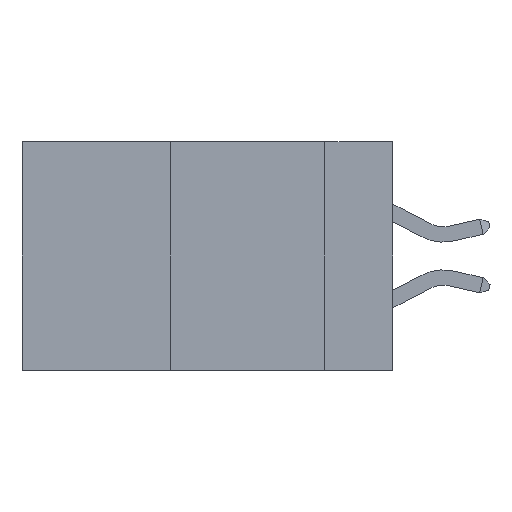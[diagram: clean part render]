
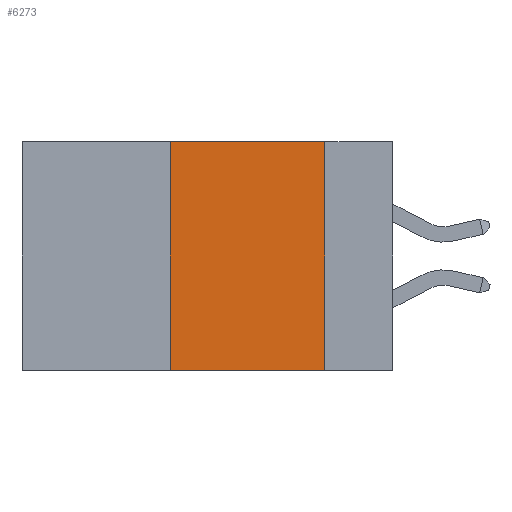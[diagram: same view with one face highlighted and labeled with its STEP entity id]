
A CAD part, left-side view. The second image highlights one B-rep face of the part: STEP entity #6273.
In plain terms, the highlighted planar face has unit normal (-1, 0, 0).
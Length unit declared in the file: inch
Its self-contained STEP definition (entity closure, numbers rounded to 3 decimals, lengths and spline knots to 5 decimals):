
#93 = EDGE_CURVE ( 'NONE', #15959, #1141, #6287, .T. ) ;
#299 = VERTEX_POINT ( 'NONE', #10447 ) ;
#703 = ORIENTED_EDGE ( 'NONE', *, *, #93, .F. ) ;
#957 = EDGE_CURVE ( 'NONE', #299, #5131, #10034, .T. ) ;
#1141 = VERTEX_POINT ( 'NONE', #5222 ) ;
#1357 = DIRECTION ( 'NONE',  ( 0., 0., 1. ) ) ;
#2706 = CARTESIAN_POINT ( 'NONE',  ( 0., 0.11, 0. ) ) ;
#3275 = DIRECTION ( 'NONE',  ( 0., -1., 0. ) ) ;
#3930 = DIRECTION ( 'NONE',  ( 0., 0., -1. ) ) ;
#3969 = CARTESIAN_POINT ( 'NONE',  ( 0., 0.6, 0. ) ) ;
#5131 = VERTEX_POINT ( 'NONE', #12251 ) ;
#5210 = VECTOR ( 'NONE', #16114, 39.37008 ) ;
#5222 = CARTESIAN_POINT ( 'NONE',  ( 0., 0.11, -0.37 ) ) ;
#5848 = VECTOR ( 'NONE', #13717, 39.37008 ) ;
#6216 = CARTESIAN_POINT ( 'NONE',  ( 0., 0.6, 0. ) ) ;
#6273 = ADVANCED_FACE ( 'NONE', ( #15174 ), #6758, .F. ) ;
#6287 = LINE ( 'NONE', #2706, #5848 ) ;
#6758 = PLANE ( 'NONE',  #11987 ) ;
#6806 = DIRECTION ( 'NONE',  ( 1., 0., 0. ) ) ;
#6867 = CARTESIAN_POINT ( 'NONE',  ( 0., 0.36, 0. ) ) ;
#7889 = EDGE_CURVE ( 'NONE', #5131, #15959, #8968, .T. ) ;
#8968 = LINE ( 'NONE', #3969, #5210 ) ;
#9175 = VECTOR ( 'NONE', #3275, 39.37008 ) ;
#10034 = LINE ( 'NONE', #6867, #14307 ) ;
#10314 = CARTESIAN_POINT ( 'NONE',  ( 0., 0.6, -0.37 ) ) ;
#10447 = CARTESIAN_POINT ( 'NONE',  ( 0., 0.36, -0.37 ) ) ;
#10464 = ORIENTED_EDGE ( 'NONE', *, *, #7889, .F. ) ;
#11151 = ORIENTED_EDGE ( 'NONE', *, *, #17406, .T. ) ;
#11692 = ORIENTED_EDGE ( 'NONE', *, *, #957, .F. ) ;
#11987 = AXIS2_PLACEMENT_3D ( 'NONE', #6216, #6806, #3930 ) ;
#12251 = CARTESIAN_POINT ( 'NONE',  ( 0., 0.36, 0. ) ) ;
#13717 = DIRECTION ( 'NONE',  ( 0., 0., -1. ) ) ;
#14307 = VECTOR ( 'NONE', #1357, 39.37008 ) ;
#15174 = FACE_OUTER_BOUND ( 'NONE', #15514, .T. ) ;
#15514 = EDGE_LOOP ( 'NONE', ( #703, #10464, #11692, #11151 ) ) ;
#15638 = CARTESIAN_POINT ( 'NONE',  ( 0., 0.11, 0. ) ) ;
#15698 = LINE ( 'NONE', #10314, #9175 ) ;
#15959 = VERTEX_POINT ( 'NONE', #15638 ) ;
#16114 = DIRECTION ( 'NONE',  ( 0., -1., 0. ) ) ;
#17406 = EDGE_CURVE ( 'NONE', #299, #1141, #15698, .T. ) ;
